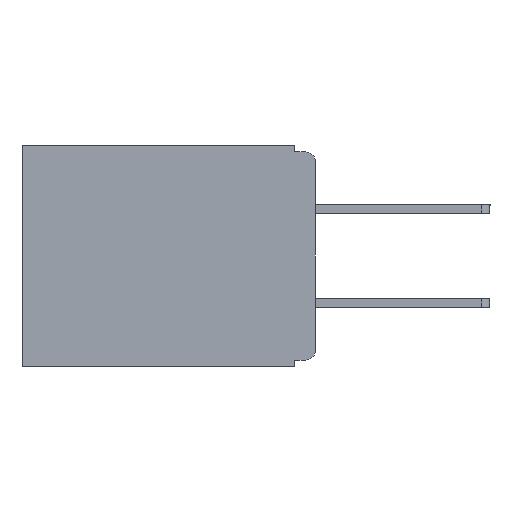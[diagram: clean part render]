
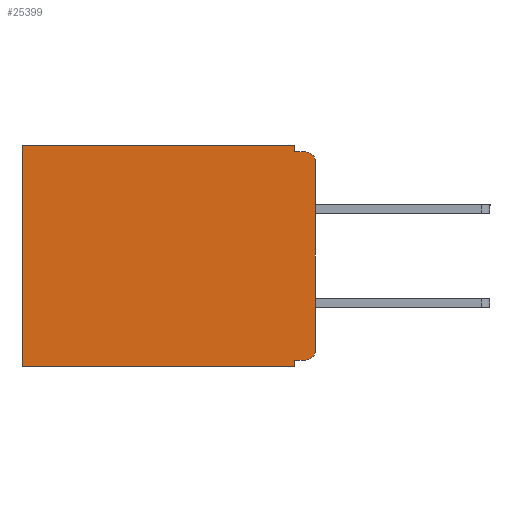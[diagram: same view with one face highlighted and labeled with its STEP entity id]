
A CAD part, left-side view. The second image highlights one B-rep face of the part: STEP entity #25399.
In plain terms, the highlighted planar face has unit normal (-1, 0, 0).
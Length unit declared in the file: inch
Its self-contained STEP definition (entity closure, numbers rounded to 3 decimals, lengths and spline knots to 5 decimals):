
#430 = CARTESIAN_POINT ( 'NONE',  ( 0.3, 0.031, 0. ) ) ;
#644 = ORIENTED_EDGE ( 'NONE', *, *, #15575, .F. ) ;
#1104 = LINE ( 'NONE', #12806, #13703 ) ;
#3370 = CARTESIAN_POINT ( 'NONE',  ( 0.3, 0.031, -0.33 ) ) ;
#4177 = ORIENTED_EDGE ( 'NONE', *, *, #17901, .T. ) ;
#4276 = VERTEX_POINT ( 'NONE', #16479 ) ;
#4607 = DIRECTION ( 'NONE',  ( 0., 1., 0. ) ) ;
#4764 = VERTEX_POINT ( 'NONE', #27661 ) ;
#4800 = ORIENTED_EDGE ( 'NONE', *, *, #13315, .F. ) ;
#5546 = DIRECTION ( 'NONE',  ( 0., 0., -1. ) ) ;
#5808 = VECTOR ( 'NONE', #17001, 39.37008 ) ;
#5871 = LINE ( 'NONE', #3370, #17502 ) ;
#6782 = VERTEX_POINT ( 'NONE', #25181 ) ;
#6968 = CARTESIAN_POINT ( 'NONE',  ( 0.3, 0.031, 0. ) ) ;
#7095 = VECTOR ( 'NONE', #23739, 39.37008 ) ;
#7294 = CARTESIAN_POINT ( 'NONE',  ( 0.3, 0.031, -0.32 ) ) ;
#7491 = ORIENTED_EDGE ( 'NONE', *, *, #13084, .T. ) ;
#7632 = DIRECTION ( 'NONE',  ( 1., 0., 0. ) ) ;
#7865 = VERTEX_POINT ( 'NONE', #18611 ) ;
#8449 = CARTESIAN_POINT ( 'NONE',  ( 0.3, 0.015, -0.305 ) ) ;
#9913 = VECTOR ( 'NONE', #5546, 39.37008 ) ;
#10972 = DIRECTION ( 'NONE',  ( 0., 0., -1. ) ) ;
#11521 = VERTEX_POINT ( 'NONE', #24809 ) ;
#12360 = CARTESIAN_POINT ( 'NONE',  ( 0.3, 0., -0.025 ) ) ;
#12806 = CARTESIAN_POINT ( 'NONE',  ( 0.3, 0., -0.33 ) ) ;
#13084 = EDGE_CURVE ( 'NONE', #11521, #30562, #16540, .T. ) ;
#13315 = EDGE_CURVE ( 'NONE', #11521, #16066, #29327, .T. ) ;
#13453 = VERTEX_POINT ( 'NONE', #12360 ) ;
#13479 = DIRECTION ( 'NONE',  ( 0., 0., -1. ) ) ;
#13703 = VECTOR ( 'NONE', #15269, 39.37008 ) ;
#13995 = DIRECTION ( 'NONE',  ( -1., 0., 0. ) ) ;
#14554 = CARTESIAN_POINT ( 'NONE',  ( 0.3, 0., -0.33 ) ) ;
#14733 = ORIENTED_EDGE ( 'NONE', *, *, #25899, .F. ) ;
#15005 = PLANE ( 'NONE',  #20167 ) ;
#15262 = DIRECTION ( 'NONE',  ( 0., 0., -1. ) ) ;
#15269 = DIRECTION ( 'NONE',  ( 0., 1., 0. ) ) ;
#15575 = EDGE_CURVE ( 'NONE', #4276, #7865, #1104, .T. ) ;
#15666 = ORIENTED_EDGE ( 'NONE', *, *, #25029, .F. ) ;
#15989 = VERTEX_POINT ( 'NONE', #6968 ) ;
#16066 = VERTEX_POINT ( 'NONE', #7294 ) ;
#16207 = LINE ( 'NONE', #25256, #22051 ) ;
#16479 = CARTESIAN_POINT ( 'NONE',  ( 0.3, 0.031, -0.33 ) ) ;
#16540 = CIRCLE ( 'NONE', #23493, 0.015 ) ;
#17001 = DIRECTION ( 'NONE',  ( 0., 0., -1. ) ) ;
#17502 = VECTOR ( 'NONE', #13479, 39.37008 ) ;
#17795 = CARTESIAN_POINT ( 'NONE',  ( 0.3, 0.437, 0. ) ) ;
#17901 = EDGE_CURVE ( 'NONE', #27352, #7865, #16207, .T. ) ;
#18476 = VECTOR ( 'NONE', #4607, 39.37008 ) ;
#18611 = CARTESIAN_POINT ( 'NONE',  ( 0.3, 0.437, -0.33 ) ) ;
#18735 = EDGE_LOOP ( 'NONE', ( #14733, #23114, #28061, #28138, #23126, #4177, #644, #15666, #4800, #7491 ) ) ;
#19350 = EDGE_CURVE ( 'NONE', #15989, #6782, #23092, .T. ) ;
#19527 = LINE ( 'NONE', #21245, #7095 ) ;
#20161 = EDGE_CURVE ( 'NONE', #6782, #4764, #19527, .T. ) ;
#20167 = AXIS2_PLACEMENT_3D ( 'NONE', #22512, #7632, #25002 ) ;
#21245 = CARTESIAN_POINT ( 'NONE',  ( 0.3, 0., -0.01 ) ) ;
#22051 = VECTOR ( 'NONE', #15262, 39.37008 ) ;
#22512 = CARTESIAN_POINT ( 'NONE',  ( 0.3, 0., -0.33 ) ) ;
#22767 = VECTOR ( 'NONE', #26657, 39.37008 ) ;
#23092 = LINE ( 'NONE', #430, #9913 ) ;
#23114 = ORIENTED_EDGE ( 'NONE', *, *, #31210, .T. ) ;
#23126 = ORIENTED_EDGE ( 'NONE', *, *, #27789, .T. ) ;
#23493 = AXIS2_PLACEMENT_3D ( 'NONE', #8449, #25824, #10972 ) ;
#23739 = DIRECTION ( 'NONE',  ( 0., -1., 0. ) ) ;
#23924 = CARTESIAN_POINT ( 'NONE',  ( 0.3, 0., -0.32 ) ) ;
#24809 = CARTESIAN_POINT ( 'NONE',  ( 0.3, 0.015, -0.32 ) ) ;
#24860 = LINE ( 'NONE', #14554, #5808 ) ;
#25002 = DIRECTION ( 'NONE',  ( 0., 0., -1. ) ) ;
#25029 = EDGE_CURVE ( 'NONE', #16066, #4276, #5871, .T. ) ;
#25181 = CARTESIAN_POINT ( 'NONE',  ( 0.3, 0.031, -0.01 ) ) ;
#25256 = CARTESIAN_POINT ( 'NONE',  ( 0.3, 0.437, -0.33 ) ) ;
#25399 = ADVANCED_FACE ( 'NONE', ( #32182 ), #15005, .F. ) ;
#25824 = DIRECTION ( 'NONE',  ( -1., 0., 0. ) ) ;
#25899 = EDGE_CURVE ( 'NONE', #13453, #30562, #24860, .T. ) ;
#25902 = LINE ( 'NONE', #26928, #18476 ) ;
#26544 = AXIS2_PLACEMENT_3D ( 'NONE', #28825, #13995, #31288 ) ;
#26657 = DIRECTION ( 'NONE',  ( 0., 1., 0. ) ) ;
#26928 = CARTESIAN_POINT ( 'NONE',  ( 0.3, 0., 0. ) ) ;
#27352 = VERTEX_POINT ( 'NONE', #17795 ) ;
#27661 = CARTESIAN_POINT ( 'NONE',  ( 0.3, 0.015, -0.01 ) ) ;
#27705 = CARTESIAN_POINT ( 'NONE',  ( 0.3, 0., -0.305 ) ) ;
#27789 = EDGE_CURVE ( 'NONE', #15989, #27352, #25902, .T. ) ;
#28061 = ORIENTED_EDGE ( 'NONE', *, *, #20161, .F. ) ;
#28138 = ORIENTED_EDGE ( 'NONE', *, *, #19350, .F. ) ;
#28330 = CIRCLE ( 'NONE', #26544, 0.015 ) ;
#28825 = CARTESIAN_POINT ( 'NONE',  ( 0.3, 0.015, -0.025 ) ) ;
#29327 = LINE ( 'NONE', #23924, #22767 ) ;
#30562 = VERTEX_POINT ( 'NONE', #27705 ) ;
#31210 = EDGE_CURVE ( 'NONE', #13453, #4764, #28330, .T. ) ;
#31288 = DIRECTION ( 'NONE',  ( 0., 0., -1. ) ) ;
#32182 = FACE_OUTER_BOUND ( 'NONE', #18735, .T. ) ;
